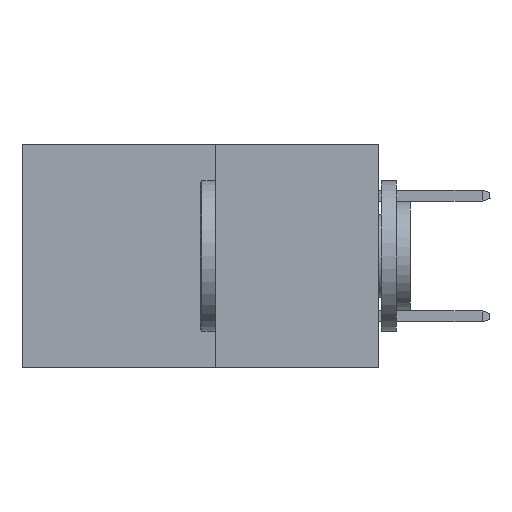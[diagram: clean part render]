
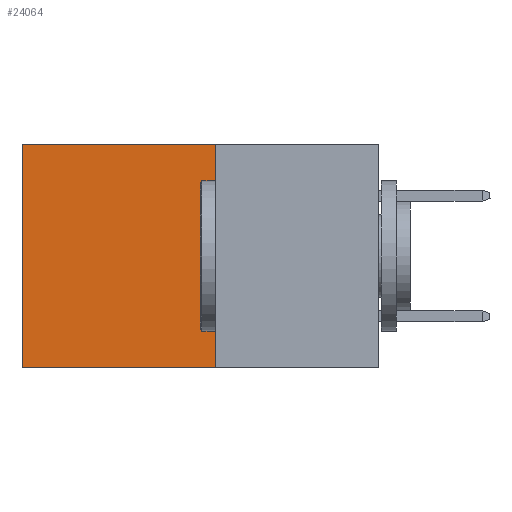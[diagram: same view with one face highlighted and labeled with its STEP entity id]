
A CAD part, left-side view. The second image highlights one B-rep face of the part: STEP entity #24064.
In plain terms, the highlighted planar face has unit normal (-1, 0, 0).
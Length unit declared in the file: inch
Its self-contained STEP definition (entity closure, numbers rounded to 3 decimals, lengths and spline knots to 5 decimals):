
#747 = VERTEX_POINT ( 'NONE', #18499 ) ;
#1423 = CARTESIAN_POINT ( 'NONE',  ( 0.277, 0.27, -0.37 ) ) ;
#1441 = VECTOR ( 'NONE', #10399, 39.37008 ) ;
#1492 = DIRECTION ( 'NONE',  ( 0., 0., -1. ) ) ;
#1790 = LINE ( 'NONE', #11614, #13234 ) ;
#2025 = EDGE_CURVE ( 'NONE', #11640, #747, #18779, .T. ) ;
#2843 = ORIENTED_EDGE ( 'NONE', *, *, #2025, .T. ) ;
#3409 = DIRECTION ( 'NONE',  ( 0., 1., 0. ) ) ;
#3439 = VECTOR ( 'NONE', #19615, 39.37008 ) ;
#6410 = CARTESIAN_POINT ( 'NONE',  ( 0.277, 0.27, 0. ) ) ;
#6874 = LINE ( 'NONE', #9653, #1441 ) ;
#8607 = EDGE_CURVE ( 'NONE', #747, #26021, #6874, .T. ) ;
#8844 = LINE ( 'NONE', #1423, #3439 ) ;
#9653 = CARTESIAN_POINT ( 'NONE',  ( 0.277, 0.59, -0.37 ) ) ;
#9774 = CARTESIAN_POINT ( 'NONE',  ( 0.277, 0.27, -0.37 ) ) ;
#10399 = DIRECTION ( 'NONE',  ( 0., 0., -1. ) ) ;
#10536 = CARTESIAN_POINT ( 'NONE',  ( 0.277, 0.27, -0.37 ) ) ;
#10982 = ORIENTED_EDGE ( 'NONE', *, *, #8607, .T. ) ;
#11614 = CARTESIAN_POINT ( 'NONE',  ( 0.277, 0.27, -0.37 ) ) ;
#11640 = VERTEX_POINT ( 'NONE', #6410 ) ;
#11790 = DIRECTION ( 'NONE',  ( 0., 0., -1. ) ) ;
#13234 = VECTOR ( 'NONE', #1492, 39.37008 ) ;
#13475 = VECTOR ( 'NONE', #3409, 39.37008 ) ;
#16358 = AXIS2_PLACEMENT_3D ( 'NONE', #9774, #23828, #11790 ) ;
#18499 = CARTESIAN_POINT ( 'NONE',  ( 0.277, 0.59, 0. ) ) ;
#18715 = ORIENTED_EDGE ( 'NONE', *, *, #19415, .F. ) ;
#18779 = LINE ( 'NONE', #21247, #13475 ) ;
#19415 = EDGE_CURVE ( 'NONE', #11640, #20289, #1790, .T. ) ;
#19615 = DIRECTION ( 'NONE',  ( 0., 1., 0. ) ) ;
#19752 = PLANE ( 'NONE',  #16358 ) ;
#19817 = EDGE_LOOP ( 'NONE', ( #10982, #21109, #18715, #2843 ) ) ;
#20289 = VERTEX_POINT ( 'NONE', #10536 ) ;
#21109 = ORIENTED_EDGE ( 'NONE', *, *, #25372, .F. ) ;
#21247 = CARTESIAN_POINT ( 'NONE',  ( 0.277, 0.27, 0. ) ) ;
#23828 = DIRECTION ( 'NONE',  ( 1., 0., 0. ) ) ;
#24064 = ADVANCED_FACE ( 'NONE', ( #24342 ), #19752, .F. ) ;
#24342 = FACE_OUTER_BOUND ( 'NONE', #19817, .T. ) ;
#25372 = EDGE_CURVE ( 'NONE', #20289, #26021, #8844, .T. ) ;
#25821 = CARTESIAN_POINT ( 'NONE',  ( 0.277, 0.59, -0.37 ) ) ;
#26021 = VERTEX_POINT ( 'NONE', #25821 ) ;
